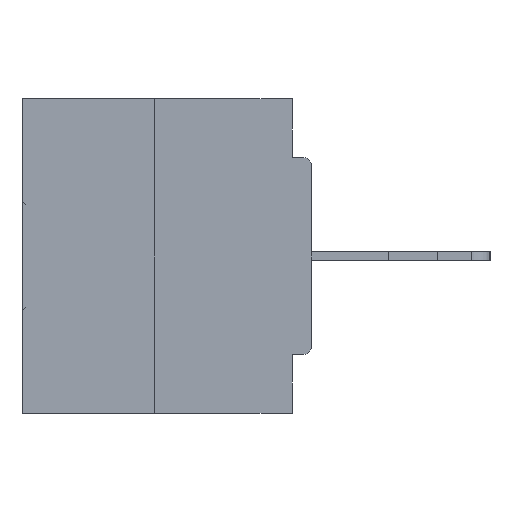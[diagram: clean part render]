
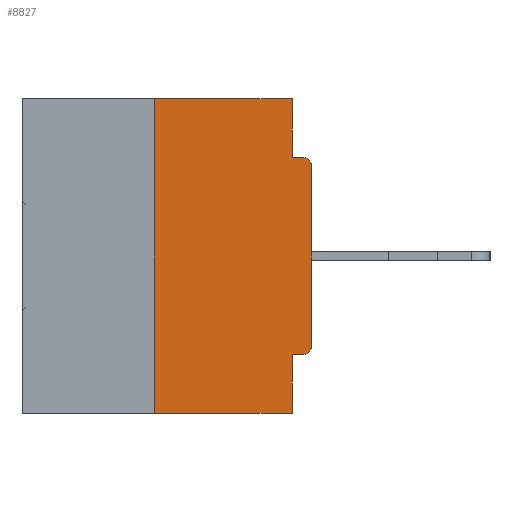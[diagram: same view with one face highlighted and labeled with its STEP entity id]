
A CAD part, left-side view. The second image highlights one B-rep face of the part: STEP entity #8827.
In plain terms, the highlighted planar face has unit normal (-1, 0, 0).
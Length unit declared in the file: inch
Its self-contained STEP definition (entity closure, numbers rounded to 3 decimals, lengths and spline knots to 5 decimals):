
#182 = CIRCLE ( 'NONE', #23892, 0.015 ) ;
#199 = VERTEX_POINT ( 'NONE', #26216 ) ;
#505 = CARTESIAN_POINT ( 'NONE',  ( 0., 0., -0.4065 ) ) ;
#717 = CARTESIAN_POINT ( 'NONE',  ( 0., 0.015, -0.4065 ) ) ;
#897 = VERTEX_POINT ( 'NONE', #4004 ) ;
#1773 = EDGE_LOOP ( 'NONE', ( #9838, #10751, #26232, #3817, #28041, #21244, #7539, #30747, #10315, #11218 ) ) ;
#2464 = VERTEX_POINT ( 'NONE', #25367 ) ;
#2728 = CARTESIAN_POINT ( 'NONE',  ( 0., 0.031, -0.4065 ) ) ;
#2939 = EDGE_CURVE ( 'NONE', #29265, #12893, #17604, .T. ) ;
#3150 = CARTESIAN_POINT ( 'NONE',  ( 0., 0.015, -0.3915 ) ) ;
#3817 = ORIENTED_EDGE ( 'NONE', *, *, #10507, .F. ) ;
#4004 = CARTESIAN_POINT ( 'NONE',  ( 0., 0.25, 0. ) ) ;
#6050 = VECTOR ( 'NONE', #24317, 39.37008 ) ;
#6105 = DIRECTION ( 'NONE',  ( 0., 0., -1. ) ) ;
#6781 = VECTOR ( 'NONE', #8118, 39.37008 ) ;
#6980 = VERTEX_POINT ( 'NONE', #20146 ) ;
#7240 = CARTESIAN_POINT ( 'NONE',  ( 0., 0.015, -0.0935 ) ) ;
#7421 = DIRECTION ( 'NONE',  ( 0., 0., -1. ) ) ;
#7539 = ORIENTED_EDGE ( 'NONE', *, *, #10614, .T. ) ;
#8118 = DIRECTION ( 'NONE',  ( 0., 0., -1. ) ) ;
#8827 = ADVANCED_FACE ( 'NONE', ( #20063 ), #28513, .F. ) ;
#9838 = ORIENTED_EDGE ( 'NONE', *, *, #23004, .F. ) ;
#9950 = VECTOR ( 'NONE', #31196, 39.37008 ) ;
#10315 = ORIENTED_EDGE ( 'NONE', *, *, #14214, .F. ) ;
#10482 = AXIS2_PLACEMENT_3D ( 'NONE', #3150, #23607, #6105 ) ;
#10507 = EDGE_CURVE ( 'NONE', #12893, #6980, #15438, .T. ) ;
#10614 = EDGE_CURVE ( 'NONE', #23242, #199, #17693, .T. ) ;
#10751 = ORIENTED_EDGE ( 'NONE', *, *, #27447, .F. ) ;
#11218 = ORIENTED_EDGE ( 'NONE', *, *, #15696, .F. ) ;
#11836 = CARTESIAN_POINT ( 'NONE',  ( 0., 0.015, -0.1085 ) ) ;
#12344 = EDGE_CURVE ( 'NONE', #29265, #23242, #20298, .T. ) ;
#12406 = VECTOR ( 'NONE', #17762, 39.37008 ) ;
#12620 = CARTESIAN_POINT ( 'NONE',  ( 0., 0.46, -0.5 ) ) ;
#12893 = VERTEX_POINT ( 'NONE', #2728 ) ;
#13117 = EDGE_CURVE ( 'NONE', #16323, #6980, #13873, .T. ) ;
#13209 = VECTOR ( 'NONE', #16415, 39.37008 ) ;
#13817 = CARTESIAN_POINT ( 'NONE',  ( 0., 0., 0. ) ) ;
#13873 = LINE ( 'NONE', #12620, #6050 ) ;
#14214 = EDGE_CURVE ( 'NONE', #21532, #32906, #28799, .T. ) ;
#14775 = DIRECTION ( 'NONE',  ( 0., 0., -1. ) ) ;
#14850 = CARTESIAN_POINT ( 'NONE',  ( 0., 0., -0.0935 ) ) ;
#15438 = LINE ( 'NONE', #27816, #29950 ) ;
#15696 = EDGE_CURVE ( 'NONE', #2464, #21532, #36787, .T. ) ;
#16323 = VERTEX_POINT ( 'NONE', #22983 ) ;
#16415 = DIRECTION ( 'NONE',  ( 0., -1., 0. ) ) ;
#16964 = DIRECTION ( 'NONE',  ( 1., 0., 0. ) ) ;
#17604 = LINE ( 'NONE', #505, #33033 ) ;
#17616 = EDGE_CURVE ( 'NONE', #199, #32906, #182, .T. ) ;
#17693 = LINE ( 'NONE', #13817, #9950 ) ;
#17762 = DIRECTION ( 'NONE',  ( 0., -1., 0. ) ) ;
#18555 = DIRECTION ( 'NONE',  ( 0., 1., 0. ) ) ;
#19375 = LINE ( 'NONE', #23559, #33872 ) ;
#20063 = FACE_OUTER_BOUND ( 'NONE', #1773, .T. ) ;
#20146 = CARTESIAN_POINT ( 'NONE',  ( 0., 0.031, -0.5 ) ) ;
#20298 = CIRCLE ( 'NONE', #10482, 0.015 ) ;
#21244 = ORIENTED_EDGE ( 'NONE', *, *, #12344, .T. ) ;
#21532 = VERTEX_POINT ( 'NONE', #32751 ) ;
#22983 = CARTESIAN_POINT ( 'NONE',  ( 0., 0.25, -0.5 ) ) ;
#23004 = EDGE_CURVE ( 'NONE', #897, #2464, #37243, .T. ) ;
#23242 = VERTEX_POINT ( 'NONE', #29091 ) ;
#23559 = CARTESIAN_POINT ( 'NONE',  ( 0., 0.25, 0. ) ) ;
#23607 = DIRECTION ( 'NONE',  ( -1., 0., 0. ) ) ;
#23892 = AXIS2_PLACEMENT_3D ( 'NONE', #11836, #32141, #14775 ) ;
#24317 = DIRECTION ( 'NONE',  ( 0., -1., 0. ) ) ;
#25367 = CARTESIAN_POINT ( 'NONE',  ( 0., 0.031, 0. ) ) ;
#25758 = AXIS2_PLACEMENT_3D ( 'NONE', #34312, #16964, #37200 ) ;
#26216 = CARTESIAN_POINT ( 'NONE',  ( 0., 0., -0.1085 ) ) ;
#26232 = ORIENTED_EDGE ( 'NONE', *, *, #13117, .T. ) ;
#27447 = EDGE_CURVE ( 'NONE', #16323, #897, #19375, .T. ) ;
#27816 = CARTESIAN_POINT ( 'NONE',  ( 0., 0.031, -0.5 ) ) ;
#28041 = ORIENTED_EDGE ( 'NONE', *, *, #2939, .F. ) ;
#28487 = CARTESIAN_POINT ( 'NONE',  ( 0., 0.031, 0. ) ) ;
#28513 = PLANE ( 'NONE',  #25758 ) ;
#28799 = LINE ( 'NONE', #14850, #12406 ) ;
#29091 = CARTESIAN_POINT ( 'NONE',  ( 0., 0., -0.3915 ) ) ;
#29265 = VERTEX_POINT ( 'NONE', #717 ) ;
#29510 = DIRECTION ( 'NONE',  ( 0., 0., 1. ) ) ;
#29950 = VECTOR ( 'NONE', #7421, 39.37008 ) ;
#30747 = ORIENTED_EDGE ( 'NONE', *, *, #17616, .T. ) ;
#30858 = CARTESIAN_POINT ( 'NONE',  ( 0., 0.46, 0. ) ) ;
#31196 = DIRECTION ( 'NONE',  ( 0., 0., 1. ) ) ;
#32141 = DIRECTION ( 'NONE',  ( -1., 0., 0. ) ) ;
#32751 = CARTESIAN_POINT ( 'NONE',  ( 0., 0.031, -0.0935 ) ) ;
#32906 = VERTEX_POINT ( 'NONE', #7240 ) ;
#33033 = VECTOR ( 'NONE', #18555, 39.37008 ) ;
#33872 = VECTOR ( 'NONE', #29510, 39.37008 ) ;
#34312 = CARTESIAN_POINT ( 'NONE',  ( 0., 0.46, 0. ) ) ;
#36787 = LINE ( 'NONE', #28487, #6781 ) ;
#37200 = DIRECTION ( 'NONE',  ( 0., 0., -1. ) ) ;
#37243 = LINE ( 'NONE', #30858, #13209 ) ;
